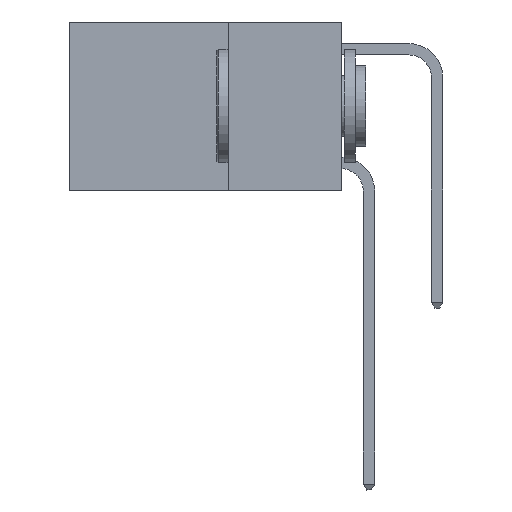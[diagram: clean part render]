
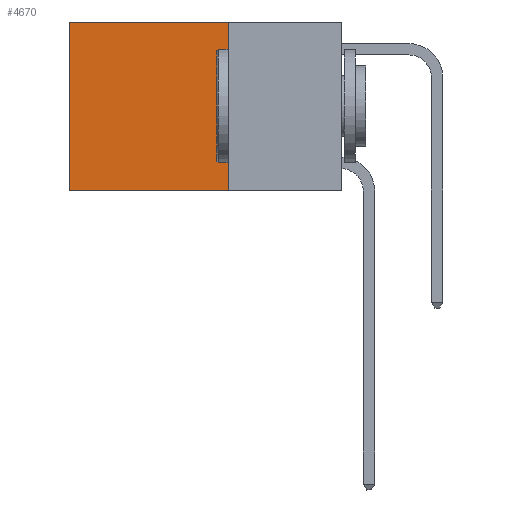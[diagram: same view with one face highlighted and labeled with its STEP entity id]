
A CAD part, left-side view. The second image highlights one B-rep face of the part: STEP entity #4670.
In plain terms, the highlighted planar face has unit normal (-1, 0, 0).
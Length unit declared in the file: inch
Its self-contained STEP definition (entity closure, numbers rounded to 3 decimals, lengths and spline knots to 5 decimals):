
#137 = DIRECTION ( 'NONE',  ( 0., 1., 0. ) ) ;
#1018 = EDGE_CURVE ( 'NONE', #6676, #1591, #10777, .T. ) ;
#1591 = VERTEX_POINT ( 'NONE', #6617 ) ;
#2564 = VECTOR ( 'NONE', #4577, 39.37008 ) ;
#3071 = FACE_OUTER_BOUND ( 'NONE', #3596, .T. ) ;
#3419 = VERTEX_POINT ( 'NONE', #4322 ) ;
#3596 = EDGE_LOOP ( 'NONE', ( #14779, #25781, #11567, #6850 ) ) ;
#4322 = CARTESIAN_POINT ( 'NONE',  ( 0.2625, 0.6, -0.37 ) ) ;
#4415 = CARTESIAN_POINT ( 'NONE',  ( 0.2625, 0.25, 0. ) ) ;
#4577 = DIRECTION ( 'NONE',  ( 0., 1., 0. ) ) ;
#4670 = ADVANCED_FACE ( 'NONE', ( #3071 ), #12932, .F. ) ;
#5625 = VECTOR ( 'NONE', #16695, 39.37008 ) ;
#6617 = CARTESIAN_POINT ( 'NONE',  ( 0.2625, 0.25, -0.37 ) ) ;
#6676 = VERTEX_POINT ( 'NONE', #4415 ) ;
#6850 = ORIENTED_EDGE ( 'NONE', *, *, #13581, .T. ) ;
#10060 = CARTESIAN_POINT ( 'NONE',  ( 0.2625, 0.6, 0. ) ) ;
#10777 = LINE ( 'NONE', #18253, #21979 ) ;
#11295 = VERTEX_POINT ( 'NONE', #21440 ) ;
#11567 = ORIENTED_EDGE ( 'NONE', *, *, #1018, .F. ) ;
#11607 = DIRECTION ( 'NONE',  ( 0., 0., -1. ) ) ;
#12932 = PLANE ( 'NONE',  #21845 ) ;
#13502 = CARTESIAN_POINT ( 'NONE',  ( 0.2625, 0.25, -0.37 ) ) ;
#13581 = EDGE_CURVE ( 'NONE', #6676, #11295, #26277, .T. ) ;
#14636 = EDGE_CURVE ( 'NONE', #11295, #3419, #23448, .T. ) ;
#14779 = ORIENTED_EDGE ( 'NONE', *, *, #14636, .T. ) ;
#15191 = DIRECTION ( 'NONE',  ( 0., 0., -1. ) ) ;
#16695 = DIRECTION ( 'NONE',  ( 0., 0., -1. ) ) ;
#17320 = CARTESIAN_POINT ( 'NONE',  ( 0.2625, 0.25, 0. ) ) ;
#18253 = CARTESIAN_POINT ( 'NONE',  ( 0.2625, 0.25, 0. ) ) ;
#19711 = LINE ( 'NONE', #13502, #20411 ) ;
#20201 = CARTESIAN_POINT ( 'NONE',  ( 0.2625, 0.25, 0. ) ) ;
#20411 = VECTOR ( 'NONE', #137, 39.37008 ) ;
#21440 = CARTESIAN_POINT ( 'NONE',  ( 0.2625, 0.6, 0. ) ) ;
#21845 = AXIS2_PLACEMENT_3D ( 'NONE', #17320, #28488, #15191 ) ;
#21979 = VECTOR ( 'NONE', #11607, 39.37008 ) ;
#23448 = LINE ( 'NONE', #10060, #5625 ) ;
#25781 = ORIENTED_EDGE ( 'NONE', *, *, #28122, .F. ) ;
#26277 = LINE ( 'NONE', #20201, #2564 ) ;
#28122 = EDGE_CURVE ( 'NONE', #1591, #3419, #19711, .T. ) ;
#28488 = DIRECTION ( 'NONE',  ( 1., 0., 0. ) ) ;
